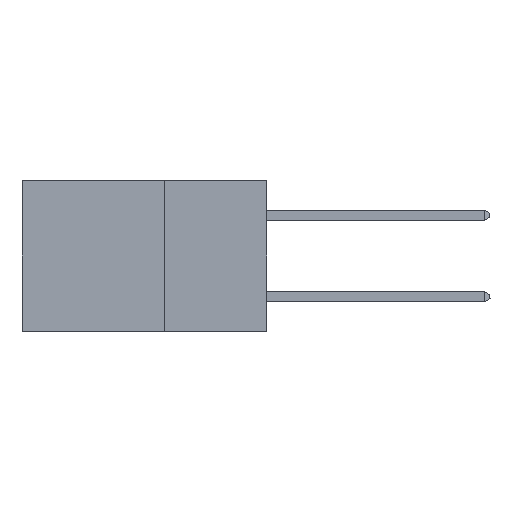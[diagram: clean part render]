
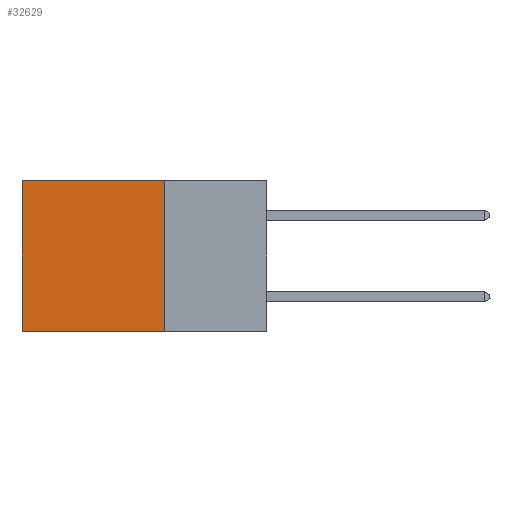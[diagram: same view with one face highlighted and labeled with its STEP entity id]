
A CAD part, left-side view. The second image highlights one B-rep face of the part: STEP entity #32629.
In plain terms, the highlighted planar face has unit normal (-1, 0, 0).
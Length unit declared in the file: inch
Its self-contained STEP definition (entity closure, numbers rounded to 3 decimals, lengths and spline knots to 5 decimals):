
#1843 = CARTESIAN_POINT ( 'NONE',  ( 0.2875, 0.6, 0. ) ) ;
#3757 = DIRECTION ( 'NONE',  ( 0., 0., -1. ) ) ;
#4322 = ORIENTED_EDGE ( 'NONE', *, *, #6597, .F. ) ;
#5356 = CARTESIAN_POINT ( 'NONE',  ( 0.2875, 0.6, 0. ) ) ;
#6122 = CARTESIAN_POINT ( 'NONE',  ( 0.2875, 0.25, 0. ) ) ;
#6597 = EDGE_CURVE ( 'NONE', #9693, #18075, #17770, .T. ) ;
#6808 = VERTEX_POINT ( 'NONE', #21309 ) ;
#9693 = VERTEX_POINT ( 'NONE', #12644 ) ;
#10795 = DIRECTION ( 'NONE',  ( 0., 0., -1. ) ) ;
#11416 = EDGE_CURVE ( 'NONE', #15538, #6808, #31089, .T. ) ;
#12644 = CARTESIAN_POINT ( 'NONE',  ( 0.2875, 0.25, 0. ) ) ;
#14224 = CARTESIAN_POINT ( 'NONE',  ( 0.2875, 0.25, 0. ) ) ;
#14417 = FACE_OUTER_BOUND ( 'NONE', #15460, .T. ) ;
#15378 = VECTOR ( 'NONE', #18234, 39.37008 ) ;
#15460 = EDGE_LOOP ( 'NONE', ( #32348, #19829, #4322, #21142 ) ) ;
#15538 = VERTEX_POINT ( 'NONE', #1843 ) ;
#16726 = EDGE_CURVE ( 'NONE', #9693, #15538, #32491, .T. ) ;
#17035 = AXIS2_PLACEMENT_3D ( 'NONE', #6122, #21387, #3757 ) ;
#17039 = EDGE_CURVE ( 'NONE', #18075, #6808, #28767, .T. ) ;
#17770 = LINE ( 'NONE', #28099, #31964 ) ;
#18075 = VERTEX_POINT ( 'NONE', #23026 ) ;
#18234 = DIRECTION ( 'NONE',  ( 0., 0., -1. ) ) ;
#19829 = ORIENTED_EDGE ( 'NONE', *, *, #17039, .F. ) ;
#21142 = ORIENTED_EDGE ( 'NONE', *, *, #16726, .T. ) ;
#21156 = DIRECTION ( 'NONE',  ( 0., 1., 0. ) ) ;
#21309 = CARTESIAN_POINT ( 'NONE',  ( 0.2875, 0.6, -0.37 ) ) ;
#21387 = DIRECTION ( 'NONE',  ( 1., 0., 0. ) ) ;
#22012 = VECTOR ( 'NONE', #24560, 39.37008 ) ;
#23026 = CARTESIAN_POINT ( 'NONE',  ( 0.2875, 0.25, -0.37 ) ) ;
#24560 = DIRECTION ( 'NONE',  ( 0., 1., 0. ) ) ;
#27122 = PLANE ( 'NONE',  #17035 ) ;
#27511 = VECTOR ( 'NONE', #21156, 39.37008 ) ;
#28099 = CARTESIAN_POINT ( 'NONE',  ( 0.2875, 0.25, 0. ) ) ;
#28767 = LINE ( 'NONE', #31617, #27511 ) ;
#31089 = LINE ( 'NONE', #5356, #15378 ) ;
#31617 = CARTESIAN_POINT ( 'NONE',  ( 0.2875, 0.25, -0.37 ) ) ;
#31964 = VECTOR ( 'NONE', #10795, 39.37008 ) ;
#32348 = ORIENTED_EDGE ( 'NONE', *, *, #11416, .T. ) ;
#32491 = LINE ( 'NONE', #14224, #22012 ) ;
#32629 = ADVANCED_FACE ( 'NONE', ( #14417 ), #27122, .F. ) ;
